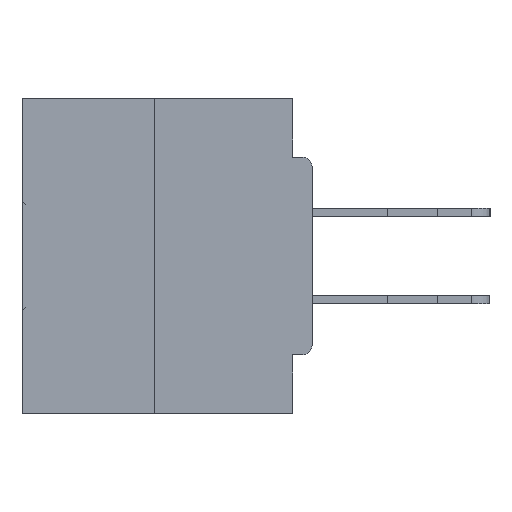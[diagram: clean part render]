
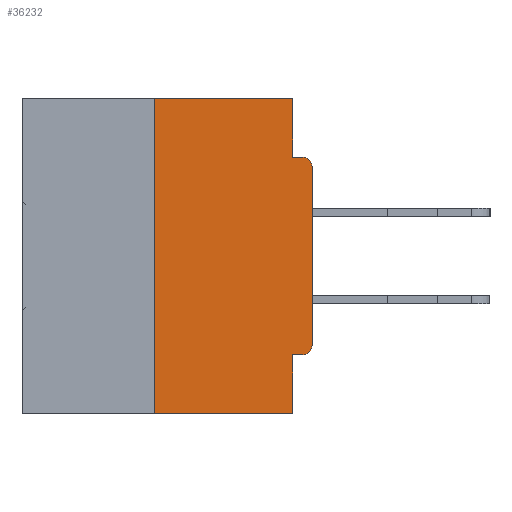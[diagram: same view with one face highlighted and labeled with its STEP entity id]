
A CAD part, left-side view. The second image highlights one B-rep face of the part: STEP entity #36232.
In plain terms, the highlighted planar face has unit normal (-1, 0, 0).
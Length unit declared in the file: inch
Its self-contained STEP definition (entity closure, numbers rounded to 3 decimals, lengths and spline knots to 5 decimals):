
#624 = CARTESIAN_POINT ( 'NONE',  ( 0., 0.031, -0.5 ) ) ;
#843 = EDGE_CURVE ( 'NONE', #35143, #22844, #35916, .T. ) ;
#936 = DIRECTION ( 'NONE',  ( 0., -1., 0. ) ) ;
#1067 = LINE ( 'NONE', #1891, #5399 ) ;
#1891 = CARTESIAN_POINT ( 'NONE',  ( 0., 0.25, 0. ) ) ;
#3319 = VECTOR ( 'NONE', #936, 39.37008 ) ;
#3608 = CARTESIAN_POINT ( 'NONE',  ( 0., 0.031, 0. ) ) ;
#4042 = EDGE_CURVE ( 'NONE', #21528, #38936, #39242, .T. ) ;
#5399 = VECTOR ( 'NONE', #8572, 39.37008 ) ;
#6163 = EDGE_CURVE ( 'NONE', #26556, #21528, #26689, .T. ) ;
#6548 = DIRECTION ( 'NONE',  ( 0., 0., 1. ) ) ;
#7769 = DIRECTION ( 'NONE',  ( 1., 0., 0. ) ) ;
#8066 = CARTESIAN_POINT ( 'NONE',  ( 0., 0.015, -0.4065 ) ) ;
#8267 = CIRCLE ( 'NONE', #21205, 0.015 ) ;
#8572 = DIRECTION ( 'NONE',  ( 0., 0., 1. ) ) ;
#10170 = EDGE_CURVE ( 'NONE', #36298, #36984, #37582, .T. ) ;
#10918 = LINE ( 'NONE', #624, #25494 ) ;
#11255 = DIRECTION ( 'NONE',  ( 0., 0., -1. ) ) ;
#11505 = CARTESIAN_POINT ( 'NONE',  ( 0., 0.25, 0. ) ) ;
#11753 = DIRECTION ( 'NONE',  ( 0., -1., 0. ) ) ;
#12771 = EDGE_CURVE ( 'NONE', #18720, #29240, #1067, .T. ) ;
#13499 = ORIENTED_EDGE ( 'NONE', *, *, #18963, .T. ) ;
#13566 = CARTESIAN_POINT ( 'NONE',  ( 0., 0.031, 0. ) ) ;
#13858 = ORIENTED_EDGE ( 'NONE', *, *, #10170, .F. ) ;
#14780 = EDGE_CURVE ( 'NONE', #18720, #44233, #31979, .T. ) ;
#15843 = DIRECTION ( 'NONE',  ( -1., 0., 0. ) ) ;
#16449 = ORIENTED_EDGE ( 'NONE', *, *, #14780, .T. ) ;
#17539 = CARTESIAN_POINT ( 'NONE',  ( 0., 0., -0.0935 ) ) ;
#17981 = ORIENTED_EDGE ( 'NONE', *, *, #44117, .T. ) ;
#18131 = ORIENTED_EDGE ( 'NONE', *, *, #843, .T. ) ;
#18199 = ORIENTED_EDGE ( 'NONE', *, *, #23414, .F. ) ;
#18347 = CARTESIAN_POINT ( 'NONE',  ( 0., 0.46, 0. ) ) ;
#18720 = VERTEX_POINT ( 'NONE', #22850 ) ;
#18963 = EDGE_CURVE ( 'NONE', #36298, #35143, #8267, .T. ) ;
#20977 = EDGE_LOOP ( 'NONE', ( #38751, #26246, #16449, #18199, #13858, #13499, #18131, #17981, #24614, #44252 ) ) ;
#21051 = DIRECTION ( 'NONE',  ( 0., -1., 0. ) ) ;
#21205 = AXIS2_PLACEMENT_3D ( 'NONE', #37635, #38086, #37492 ) ;
#21293 = DIRECTION ( 'NONE',  ( 0., 0., -1. ) ) ;
#21315 = VECTOR ( 'NONE', #6548, 39.37008 ) ;
#21528 = VERTEX_POINT ( 'NONE', #32050 ) ;
#22844 = VERTEX_POINT ( 'NONE', #42031 ) ;
#22850 = CARTESIAN_POINT ( 'NONE',  ( 0., 0.25, -0.5 ) ) ;
#23414 = EDGE_CURVE ( 'NONE', #36984, #44233, #10918, .T. ) ;
#24614 = ORIENTED_EDGE ( 'NONE', *, *, #4042, .F. ) ;
#25067 = CARTESIAN_POINT ( 'NONE',  ( 0., 0., -0.3915 ) ) ;
#25084 = LINE ( 'NONE', #42590, #43992 ) ;
#25494 = VECTOR ( 'NONE', #28432, 39.37008 ) ;
#25847 = CARTESIAN_POINT ( 'NONE',  ( 0., 0.031, -0.5 ) ) ;
#26231 = VECTOR ( 'NONE', #30369, 39.37008 ) ;
#26246 = ORIENTED_EDGE ( 'NONE', *, *, #12771, .F. ) ;
#26302 = CARTESIAN_POINT ( 'NONE',  ( 0., 0.015, -0.1085 ) ) ;
#26556 = VERTEX_POINT ( 'NONE', #13566 ) ;
#26689 = LINE ( 'NONE', #3608, #42878 ) ;
#28333 = FACE_OUTER_BOUND ( 'NONE', #20977, .T. ) ;
#28432 = DIRECTION ( 'NONE',  ( 0., 0., -1. ) ) ;
#29240 = VERTEX_POINT ( 'NONE', #11505 ) ;
#29446 = CIRCLE ( 'NONE', #36606, 0.015 ) ;
#30369 = DIRECTION ( 'NONE',  ( 0., 1., 0. ) ) ;
#31550 = EDGE_CURVE ( 'NONE', #29240, #26556, #25084, .T. ) ;
#31979 = LINE ( 'NONE', #35255, #3319 ) ;
#32050 = CARTESIAN_POINT ( 'NONE',  ( 0., 0.031, -0.0935 ) ) ;
#33869 = CARTESIAN_POINT ( 'NONE',  ( 0., 0., -0.4065 ) ) ;
#35143 = VERTEX_POINT ( 'NONE', #25067 ) ;
#35255 = CARTESIAN_POINT ( 'NONE',  ( 0., 0.46, -0.5 ) ) ;
#35889 = PLANE ( 'NONE',  #39812 ) ;
#35916 = LINE ( 'NONE', #36490, #21315 ) ;
#36232 = ADVANCED_FACE ( 'NONE', ( #28333 ), #35889, .F. ) ;
#36298 = VERTEX_POINT ( 'NONE', #8066 ) ;
#36490 = CARTESIAN_POINT ( 'NONE',  ( 0., 0., 0. ) ) ;
#36606 = AXIS2_PLACEMENT_3D ( 'NONE', #26302, #15843, #43052 ) ;
#36984 = VERTEX_POINT ( 'NONE', #40519 ) ;
#37492 = DIRECTION ( 'NONE',  ( 0., 0., -1. ) ) ;
#37582 = LINE ( 'NONE', #33869, #26231 ) ;
#37635 = CARTESIAN_POINT ( 'NONE',  ( 0., 0.015, -0.3915 ) ) ;
#38086 = DIRECTION ( 'NONE',  ( -1., 0., 0. ) ) ;
#38169 = CARTESIAN_POINT ( 'NONE',  ( 0., 0.015, -0.0935 ) ) ;
#38751 = ORIENTED_EDGE ( 'NONE', *, *, #31550, .F. ) ;
#38936 = VERTEX_POINT ( 'NONE', #38169 ) ;
#39242 = LINE ( 'NONE', #17539, #44079 ) ;
#39812 = AXIS2_PLACEMENT_3D ( 'NONE', #18347, #7769, #11255 ) ;
#40519 = CARTESIAN_POINT ( 'NONE',  ( 0., 0.031, -0.4065 ) ) ;
#42031 = CARTESIAN_POINT ( 'NONE',  ( 0., 0., -0.1085 ) ) ;
#42590 = CARTESIAN_POINT ( 'NONE',  ( 0., 0.46, 0. ) ) ;
#42878 = VECTOR ( 'NONE', #21293, 39.37008 ) ;
#43052 = DIRECTION ( 'NONE',  ( 0., 0., -1. ) ) ;
#43992 = VECTOR ( 'NONE', #11753, 39.37008 ) ;
#44079 = VECTOR ( 'NONE', #21051, 39.37008 ) ;
#44117 = EDGE_CURVE ( 'NONE', #22844, #38936, #29446, .T. ) ;
#44233 = VERTEX_POINT ( 'NONE', #25847 ) ;
#44252 = ORIENTED_EDGE ( 'NONE', *, *, #6163, .F. ) ;
